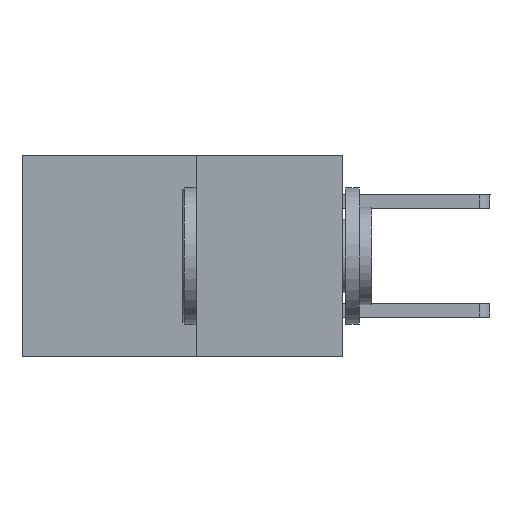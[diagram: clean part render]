
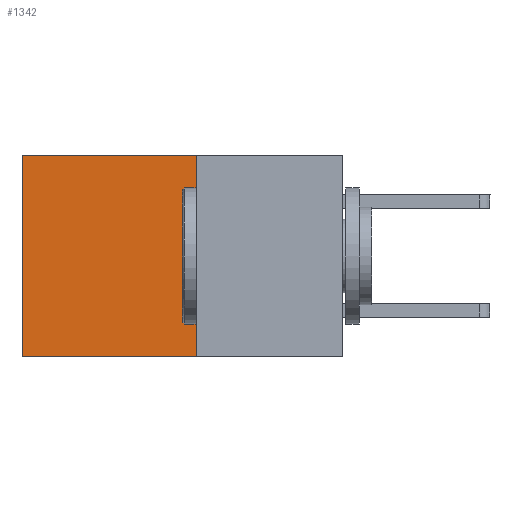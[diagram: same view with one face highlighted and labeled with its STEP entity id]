
A CAD part, left-side view. The second image highlights one B-rep face of the part: STEP entity #1342.
In plain terms, the highlighted planar face has unit normal (-1, 0, 0).
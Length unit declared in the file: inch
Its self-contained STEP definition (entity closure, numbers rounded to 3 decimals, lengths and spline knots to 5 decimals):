
#143 = ORIENTED_EDGE ( 'NONE', *, *, #9821, .F. ) ;
#175 = DIRECTION ( 'NONE',  ( 1., 0., 0. ) ) ;
#174 = LINE ( 'NONE', #3312, #7661 ) ;
#181 = DIRECTION ( 'NONE',  ( 0., 0., -1. ) ) ;
#423 = VECTOR ( 'NONE', #9124, 39.37008 ) ;
#424 = CARTESIAN_POINT ( 'NONE',  ( 0.277, 0.59, -0.37 ) ) ;
#605 = VECTOR ( 'NONE', #181, 39.37008 ) ;
#825 = CARTESIAN_POINT ( 'NONE',  ( 0.277, 0.27, -0.37 ) ) ;
#871 = AXIS2_PLACEMENT_3D ( 'NONE', #825, #175, #6426 ) ;
#1262 = CARTESIAN_POINT ( 'NONE',  ( 0.277, 0.27, 0. ) ) ;
#1342 = ADVANCED_FACE ( 'NONE', ( #4764 ), #1745, .F. ) ;
#1745 = PLANE ( 'NONE',  #871 ) ;
#2001 = VERTEX_POINT ( 'NONE', #8145 ) ;
#2558 = DIRECTION ( 'NONE',  ( 0., 0., -1. ) ) ;
#2627 = VECTOR ( 'NONE', #2678, 39.37008 ) ;
#2678 = DIRECTION ( 'NONE',  ( 0., 1., 0. ) ) ;
#2846 = CARTESIAN_POINT ( 'NONE',  ( 0.277, 0.59, 0. ) ) ;
#3312 = CARTESIAN_POINT ( 'NONE',  ( 0.277, 0.27, -0.37 ) ) ;
#3557 = ORIENTED_EDGE ( 'NONE', *, *, #5455, .T. ) ;
#3904 = ORIENTED_EDGE ( 'NONE', *, *, #4320, .T. ) ;
#4320 = EDGE_CURVE ( 'NONE', #9482, #4341, #6726, .T. ) ;
#4341 = VERTEX_POINT ( 'NONE', #2846 ) ;
#4764 = FACE_OUTER_BOUND ( 'NONE', #9151, .T. ) ;
#5317 = CARTESIAN_POINT ( 'NONE',  ( 0.277, 0.27, 0. ) ) ;
#5455 = EDGE_CURVE ( 'NONE', #4341, #5643, #7692, .T. ) ;
#5643 = VERTEX_POINT ( 'NONE', #424 ) ;
#5743 = CARTESIAN_POINT ( 'NONE',  ( 0.277, 0.27, -0.37 ) ) ;
#5769 = ORIENTED_EDGE ( 'NONE', *, *, #7538, .F. ) ;
#6426 = DIRECTION ( 'NONE',  ( 0., 0., -1. ) ) ;
#6726 = LINE ( 'NONE', #1262, #423 ) ;
#7237 = CARTESIAN_POINT ( 'NONE',  ( 0.277, 0.59, -0.37 ) ) ;
#7538 = EDGE_CURVE ( 'NONE', #2001, #5643, #9563, .T. ) ;
#7661 = VECTOR ( 'NONE', #2558, 39.37008 ) ;
#7692 = LINE ( 'NONE', #7237, #605 ) ;
#8145 = CARTESIAN_POINT ( 'NONE',  ( 0.277, 0.27, -0.37 ) ) ;
#9124 = DIRECTION ( 'NONE',  ( 0., 1., 0. ) ) ;
#9151 = EDGE_LOOP ( 'NONE', ( #3557, #5769, #143, #3904 ) ) ;
#9482 = VERTEX_POINT ( 'NONE', #5317 ) ;
#9563 = LINE ( 'NONE', #5743, #2627 ) ;
#9821 = EDGE_CURVE ( 'NONE', #9482, #2001, #174, .T. ) ;
